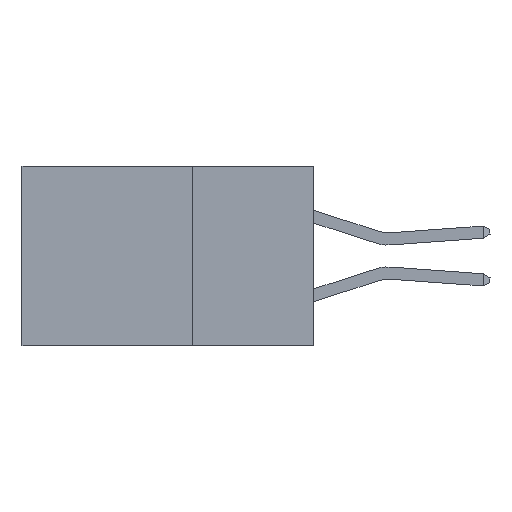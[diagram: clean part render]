
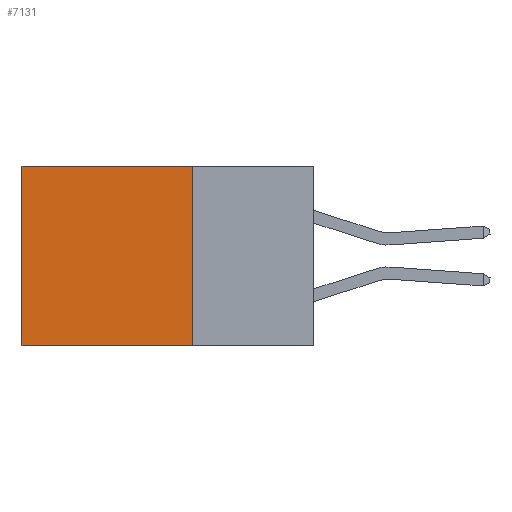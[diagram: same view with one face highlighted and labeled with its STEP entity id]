
A CAD part, left-side view. The second image highlights one B-rep face of the part: STEP entity #7131.
In plain terms, the highlighted planar face has unit normal (-1, 0, 0).
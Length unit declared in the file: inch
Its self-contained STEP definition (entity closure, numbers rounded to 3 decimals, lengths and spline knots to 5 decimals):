
#479 = CARTESIAN_POINT ( 'NONE',  ( 0.2875, 0.25, 0. ) ) ;
#955 = PLANE ( 'NONE',  #2424 ) ;
#2424 = AXIS2_PLACEMENT_3D ( 'NONE', #33628, #30200, #18636 ) ;
#6159 = ORIENTED_EDGE ( 'NONE', *, *, #29764, .F. ) ;
#7131 = ADVANCED_FACE ( 'NONE', ( #29097 ), #955, .F. ) ;
#9304 = ORIENTED_EDGE ( 'NONE', *, *, #25090, .T. ) ;
#10367 = VERTEX_POINT ( 'NONE', #37823 ) ;
#11073 = CARTESIAN_POINT ( 'NONE',  ( 0.2875, 0.6, 0. ) ) ;
#12286 = CARTESIAN_POINT ( 'NONE',  ( 0.2875, 0.6, 0. ) ) ;
#12721 = VECTOR ( 'NONE', #27415, 39.37008 ) ;
#13849 = VECTOR ( 'NONE', #35507, 39.37008 ) ;
#16571 = VERTEX_POINT ( 'NONE', #11073 ) ;
#18636 = DIRECTION ( 'NONE',  ( 0., 0., -1. ) ) ;
#20666 = EDGE_CURVE ( 'NONE', #25227, #27996, #32585, .T. ) ;
#22616 = LINE ( 'NONE', #12286, #13849 ) ;
#23235 = DIRECTION ( 'NONE',  ( 0., 1., 0. ) ) ;
#25090 = EDGE_CURVE ( 'NONE', #16571, #10367, #22616, .T. ) ;
#25227 = VERTEX_POINT ( 'NONE', #30633 ) ;
#25853 = ORIENTED_EDGE ( 'NONE', *, *, #20666, .F. ) ;
#27415 = DIRECTION ( 'NONE',  ( 0., 0., -1. ) ) ;
#27996 = VERTEX_POINT ( 'NONE', #36093 ) ;
#28388 = VECTOR ( 'NONE', #29080, 39.37008 ) ;
#28854 = LINE ( 'NONE', #34860, #28388 ) ;
#29080 = DIRECTION ( 'NONE',  ( 0., 1., 0. ) ) ;
#29097 = FACE_OUTER_BOUND ( 'NONE', #33574, .T. ) ;
#29422 = CARTESIAN_POINT ( 'NONE',  ( 0.2875, 0.25, -0.37 ) ) ;
#29764 = EDGE_CURVE ( 'NONE', #27996, #10367, #31381, .T. ) ;
#30200 = DIRECTION ( 'NONE',  ( 1., 0., 0. ) ) ;
#30633 = CARTESIAN_POINT ( 'NONE',  ( 0.2875, 0.25, 0. ) ) ;
#31381 = LINE ( 'NONE', #29422, #37365 ) ;
#32585 = LINE ( 'NONE', #479, #12721 ) ;
#33574 = EDGE_LOOP ( 'NONE', ( #9304, #6159, #25853, #37333 ) ) ;
#33628 = CARTESIAN_POINT ( 'NONE',  ( 0.2875, 0.25, 0. ) ) ;
#33957 = EDGE_CURVE ( 'NONE', #25227, #16571, #28854, .T. ) ;
#34860 = CARTESIAN_POINT ( 'NONE',  ( 0.2875, 0.25, 0. ) ) ;
#35507 = DIRECTION ( 'NONE',  ( 0., 0., -1. ) ) ;
#36093 = CARTESIAN_POINT ( 'NONE',  ( 0.2875, 0.25, -0.37 ) ) ;
#37333 = ORIENTED_EDGE ( 'NONE', *, *, #33957, .T. ) ;
#37365 = VECTOR ( 'NONE', #23235, 39.37008 ) ;
#37823 = CARTESIAN_POINT ( 'NONE',  ( 0.2875, 0.6, -0.37 ) ) ;
